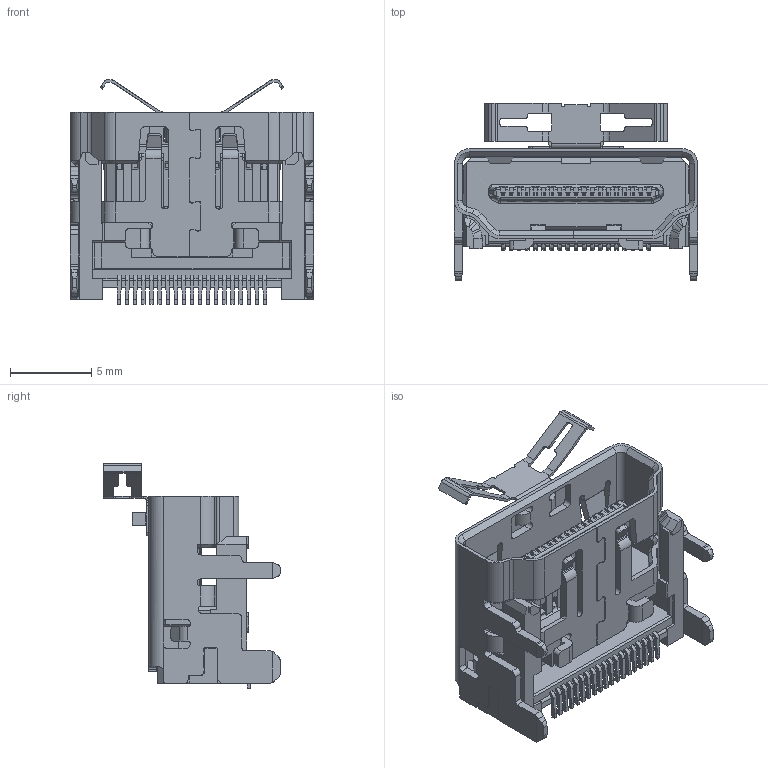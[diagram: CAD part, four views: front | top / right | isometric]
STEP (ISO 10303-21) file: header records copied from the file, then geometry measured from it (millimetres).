
FILE_DESCRIPTION (( 'STEP AP214' ), '1' );
FILE_NAME ('694D119E164-011.STEP', '2021-01-13T16:06:09', ( '' ), ( '' ), 'SwSTEP 2.0', 'SolidWorks 2020', '' );
FILE_SCHEMA (( 'AUTOMOTIVE_DESIGN' ));
Length unit declared in the file: millimetre
Products named in the file (5): EMI 694D119EX64-011; Insulator 694D119EX64-011; Contacts 694D119EX64-011; Shell 694D119EX64-011; 694D119E164-011
Assembly tree (4 placements, depth 2):
  694D119E164-011
    Insulator 694D119EX64-011
    Contacts 694D119EX64-011
    Shell 694D119EX64-011
    EMI 694D119EX64-011
Bounding box: 15 x 10.93 x 13.87 mm (x, y, z)
Volume: 452.9 mm3; surface area: 1904.9 mm2
Topology: 22 solids, 22 shells, 3527 faces, 10325 edges, 6730 vertices
Faces by surface type: plane 2264, cylinder 1188, bspline 39, cone 27, torus 5, sphere 4
Entity records: 117819 total; most frequent: CARTESIAN_POINT 23197, ORIENTED_EDGE 20642, DIRECTION 18896, EDGE_CURVE 10321, VECTOR 7230, LINE 7230, VERTEX_POINT 6729, AXIS2_PLACEMENT_3D 5833
